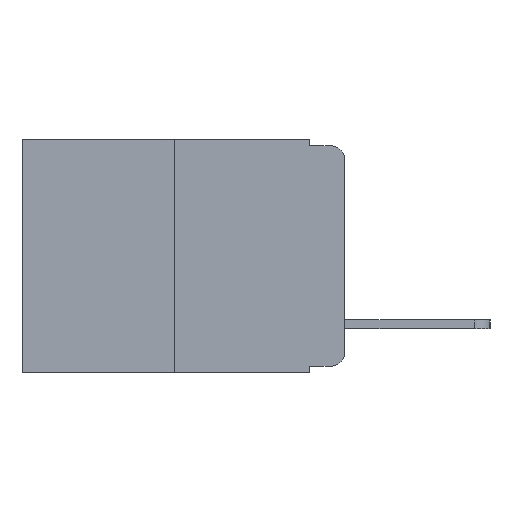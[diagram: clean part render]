
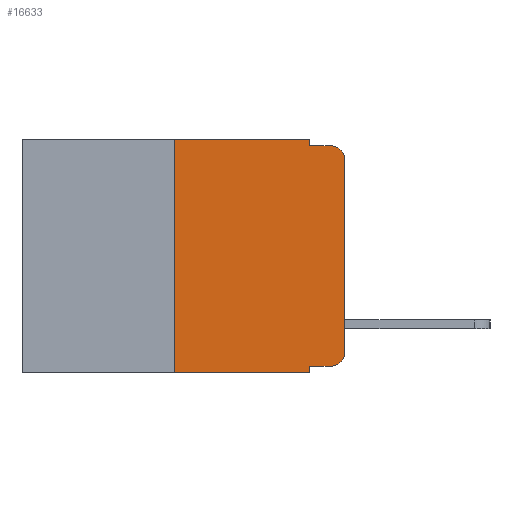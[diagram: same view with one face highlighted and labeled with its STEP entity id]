
A CAD part, left-side view. The second image highlights one B-rep face of the part: STEP entity #16633.
In plain terms, the highlighted planar face has unit normal (-1, 0, 0).
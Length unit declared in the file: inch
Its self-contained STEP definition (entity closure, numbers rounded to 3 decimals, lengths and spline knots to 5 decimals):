
#367 = ORIENTED_EDGE ( 'NONE', *, *, #5531, .T. ) ;
#462 = DIRECTION ( 'NONE',  ( 0., 0., -1. ) ) ;
#705 = ORIENTED_EDGE ( 'NONE', *, *, #1075, .F. ) ;
#767 = ORIENTED_EDGE ( 'NONE', *, *, #6533, .T. ) ;
#1075 = EDGE_CURVE ( 'NONE', #7516, #3826, #15072, .T. ) ;
#1277 = ORIENTED_EDGE ( 'NONE', *, *, #16053, .T. ) ;
#1278 = CARTESIAN_POINT ( 'NONE',  ( 0., 0.473, 0. ) ) ;
#1551 = CARTESIAN_POINT ( 'NONE',  ( 0., 0.051, 0. ) ) ;
#1602 = VECTOR ( 'NONE', #3738, 39.37008 ) ;
#1721 = LINE ( 'NONE', #6407, #12684 ) ;
#1875 = ORIENTED_EDGE ( 'NONE', *, *, #8066, .F. ) ;
#1898 = ORIENTED_EDGE ( 'NONE', *, *, #6879, .T. ) ;
#2178 = LINE ( 'NONE', #11063, #1602 ) ;
#2271 = LINE ( 'NONE', #6434, #9845 ) ;
#2390 = VERTEX_POINT ( 'NONE', #6751 ) ;
#2483 = CARTESIAN_POINT ( 'NONE',  ( 0., 0.02, -0.03 ) ) ;
#3000 = DIRECTION ( 'NONE',  ( 0., 0., -1. ) ) ;
#3089 = LINE ( 'NONE', #7860, #14237 ) ;
#3312 = ORIENTED_EDGE ( 'NONE', *, *, #10911, .F. ) ;
#3566 = ORIENTED_EDGE ( 'NONE', *, *, #18936, .T. ) ;
#3738 = DIRECTION ( 'NONE',  ( 0., 0., 1. ) ) ;
#3814 = LINE ( 'NONE', #9580, #14892 ) ;
#3826 = VERTEX_POINT ( 'NONE', #8755 ) ;
#3919 = VERTEX_POINT ( 'NONE', #8093 ) ;
#4025 = EDGE_CURVE ( 'NONE', #6548, #2390, #7634, .T. ) ;
#4097 = DIRECTION ( 'NONE',  ( 0., 0., -1. ) ) ;
#4199 = CARTESIAN_POINT ( 'NONE',  ( 0., 0.02, -0.333 ) ) ;
#4275 = VERTEX_POINT ( 'NONE', #4199 ) ;
#4622 = VERTEX_POINT ( 'NONE', #15742 ) ;
#4655 = VECTOR ( 'NONE', #18781, 39.37008 ) ;
#5531 = EDGE_CURVE ( 'NONE', #7854, #3919, #3814, .T. ) ;
#6345 = DIRECTION ( 'NONE',  ( 0., -1., 0. ) ) ;
#6407 = CARTESIAN_POINT ( 'NONE',  ( 0., 0.051, -0.333 ) ) ;
#6434 = CARTESIAN_POINT ( 'NONE',  ( 0., 0.473, 0. ) ) ;
#6498 = DIRECTION ( 'NONE',  ( -1., 0., 0. ) ) ;
#6533 = EDGE_CURVE ( 'NONE', #3919, #18635, #18790, .T. ) ;
#6548 = VERTEX_POINT ( 'NONE', #14188 ) ;
#6751 = CARTESIAN_POINT ( 'NONE',  ( 0., 0.051, -0.01 ) ) ;
#6879 = EDGE_CURVE ( 'NONE', #4622, #3826, #3089, .T. ) ;
#7269 = CIRCLE ( 'NONE', #10968, 0.02 ) ;
#7354 = CARTESIAN_POINT ( 'NONE',  ( 0., 0.051, -0.01 ) ) ;
#7516 = VERTEX_POINT ( 'NONE', #12156 ) ;
#7634 = LINE ( 'NONE', #1551, #18555 ) ;
#7854 = VERTEX_POINT ( 'NONE', #11710 ) ;
#7860 = CARTESIAN_POINT ( 'NONE',  ( 0., 0.473, -0.343 ) ) ;
#7947 = DIRECTION ( 'NONE',  ( 0., -1., 0. ) ) ;
#8066 = EDGE_CURVE ( 'NONE', #10164, #6548, #2271, .T. ) ;
#8093 = CARTESIAN_POINT ( 'NONE',  ( 0., 0., -0.03 ) ) ;
#8641 = LINE ( 'NONE', #7354, #4655 ) ;
#8755 = CARTESIAN_POINT ( 'NONE',  ( 0., 0.051, -0.343 ) ) ;
#8964 = ORIENTED_EDGE ( 'NONE', *, *, #11263, .F. ) ;
#9580 = CARTESIAN_POINT ( 'NONE',  ( 0., 0., 0. ) ) ;
#9845 = VECTOR ( 'NONE', #7947, 39.37008 ) ;
#10164 = VERTEX_POINT ( 'NONE', #18050 ) ;
#10206 = EDGE_LOOP ( 'NONE', ( #367, #767, #8964, #16463, #1875, #3312, #1898, #705, #1277, #3566 ) ) ;
#10322 = CARTESIAN_POINT ( 'NONE',  ( 0., 0.02, -0.01 ) ) ;
#10911 = EDGE_CURVE ( 'NONE', #4622, #10164, #2178, .T. ) ;
#10968 = AXIS2_PLACEMENT_3D ( 'NONE', #15046, #6498, #16555 ) ;
#10983 = DIRECTION ( 'NONE',  ( 0., 0., 1. ) ) ;
#11063 = CARTESIAN_POINT ( 'NONE',  ( 0., 0.25, 0. ) ) ;
#11263 = EDGE_CURVE ( 'NONE', #2390, #18635, #8641, .T. ) ;
#11324 = VECTOR ( 'NONE', #462, 39.37008 ) ;
#11710 = CARTESIAN_POINT ( 'NONE',  ( 0., 0., -0.313 ) ) ;
#11824 = DIRECTION ( 'NONE',  ( 1., 0., 0. ) ) ;
#12156 = CARTESIAN_POINT ( 'NONE',  ( 0., 0.051, -0.333 ) ) ;
#12684 = VECTOR ( 'NONE', #14938, 39.37008 ) ;
#12803 = DIRECTION ( 'NONE',  ( -1., 0., 0. ) ) ;
#13925 = AXIS2_PLACEMENT_3D ( 'NONE', #2483, #12803, #4097 ) ;
#14188 = CARTESIAN_POINT ( 'NONE',  ( 0., 0.051, 0. ) ) ;
#14237 = VECTOR ( 'NONE', #6345, 39.37008 ) ;
#14892 = VECTOR ( 'NONE', #10983, 39.37008 ) ;
#14938 = DIRECTION ( 'NONE',  ( 0., -1., 0. ) ) ;
#15046 = CARTESIAN_POINT ( 'NONE',  ( 0., 0.02, -0.313 ) ) ;
#15072 = LINE ( 'NONE', #16831, #11324 ) ;
#15184 = DIRECTION ( 'NONE',  ( 0., 0., -1. ) ) ;
#15742 = CARTESIAN_POINT ( 'NONE',  ( 0., 0.25, -0.343 ) ) ;
#16053 = EDGE_CURVE ( 'NONE', #7516, #4275, #1721, .T. ) ;
#16463 = ORIENTED_EDGE ( 'NONE', *, *, #4025, .F. ) ;
#16555 = DIRECTION ( 'NONE',  ( 0., 0., -1. ) ) ;
#16633 = ADVANCED_FACE ( 'NONE', ( #18921 ), #18951, .F. ) ;
#16831 = CARTESIAN_POINT ( 'NONE',  ( 0., 0.051, 0. ) ) ;
#18050 = CARTESIAN_POINT ( 'NONE',  ( 0., 0.25, 0. ) ) ;
#18077 = AXIS2_PLACEMENT_3D ( 'NONE', #1278, #11824, #3000 ) ;
#18555 = VECTOR ( 'NONE', #15184, 39.37008 ) ;
#18635 = VERTEX_POINT ( 'NONE', #10322 ) ;
#18781 = DIRECTION ( 'NONE',  ( 0., -1., 0. ) ) ;
#18790 = CIRCLE ( 'NONE', #13925, 0.02 ) ;
#18921 = FACE_OUTER_BOUND ( 'NONE', #10206, .T. ) ;
#18936 = EDGE_CURVE ( 'NONE', #4275, #7854, #7269, .T. ) ;
#18951 = PLANE ( 'NONE',  #18077 ) ;
